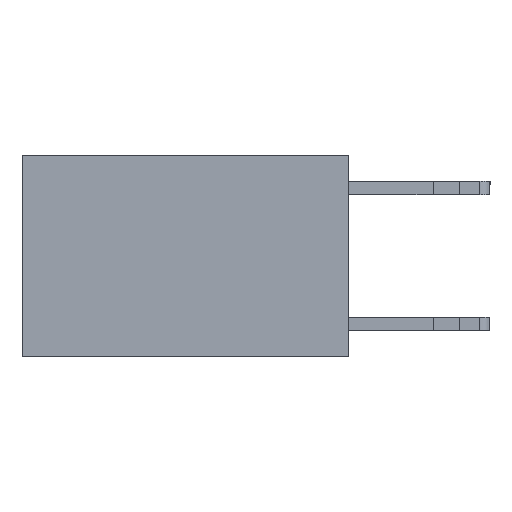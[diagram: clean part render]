
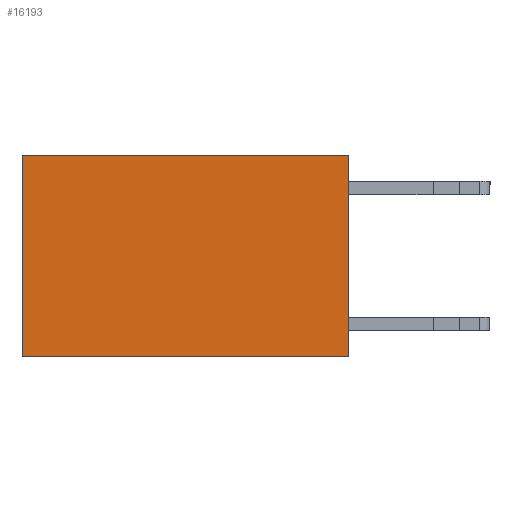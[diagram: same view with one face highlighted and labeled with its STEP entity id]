
A CAD part, left-side view. The second image highlights one B-rep face of the part: STEP entity #16193.
In plain terms, the highlighted planar face has unit normal (-1, 0, 0).
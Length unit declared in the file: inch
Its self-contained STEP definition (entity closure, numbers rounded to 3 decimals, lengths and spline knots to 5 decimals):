
#181 = FACE_OUTER_BOUND ( 'NONE', #7099, .T. ) ;
#214 = DIRECTION ( 'NONE',  ( 0., 1., 0. ) ) ;
#732 = VERTEX_POINT ( 'NONE', #15898 ) ;
#791 = EDGE_CURVE ( 'NONE', #1313, #732, #14803, .T. ) ;
#1313 = VERTEX_POINT ( 'NONE', #6391 ) ;
#1905 = CARTESIAN_POINT ( 'NONE',  ( 0.2625, 0., -0.37 ) ) ;
#4133 = DIRECTION ( 'NONE',  ( 0., 0., -1. ) ) ;
#4247 = LINE ( 'NONE', #9738, #13592 ) ;
#4595 = VECTOR ( 'NONE', #4133, 39.37008 ) ;
#5640 = PLANE ( 'NONE',  #14973 ) ;
#5733 = CARTESIAN_POINT ( 'NONE',  ( 0.2625, 0., 0. ) ) ;
#6015 = EDGE_CURVE ( 'NONE', #7714, #14525, #10716, .T. ) ;
#6265 = EDGE_CURVE ( 'NONE', #7714, #1313, #6900, .T. ) ;
#6391 = CARTESIAN_POINT ( 'NONE',  ( 0.2625, 0.6, 0. ) ) ;
#6900 = LINE ( 'NONE', #12488, #12908 ) ;
#7099 = EDGE_LOOP ( 'NONE', ( #16172, #9218, #14321, #10500 ) ) ;
#7173 = DIRECTION ( 'NONE',  ( 0., 0., -1. ) ) ;
#7268 = DIRECTION ( 'NONE',  ( 1., 0., 0. ) ) ;
#7714 = VERTEX_POINT ( 'NONE', #5733 ) ;
#8097 = CARTESIAN_POINT ( 'NONE',  ( 0.2625, 0.6, 0. ) ) ;
#9218 = ORIENTED_EDGE ( 'NONE', *, *, #10481, .F. ) ;
#9738 = CARTESIAN_POINT ( 'NONE',  ( 0.2625, 0., -0.37 ) ) ;
#10481 = EDGE_CURVE ( 'NONE', #14525, #732, #4247, .T. ) ;
#10500 = ORIENTED_EDGE ( 'NONE', *, *, #6265, .T. ) ;
#10656 = DIRECTION ( 'NONE',  ( 0., 0., -1. ) ) ;
#10716 = LINE ( 'NONE', #17465, #4595 ) ;
#12488 = CARTESIAN_POINT ( 'NONE',  ( 0.2625, 0., 0. ) ) ;
#12908 = VECTOR ( 'NONE', #16815, 39.37008 ) ;
#13592 = VECTOR ( 'NONE', #214, 39.37008 ) ;
#14321 = ORIENTED_EDGE ( 'NONE', *, *, #6015, .F. ) ;
#14525 = VERTEX_POINT ( 'NONE', #1905 ) ;
#14803 = LINE ( 'NONE', #8097, #16113 ) ;
#14973 = AXIS2_PLACEMENT_3D ( 'NONE', #16650, #7268, #7173 ) ;
#15898 = CARTESIAN_POINT ( 'NONE',  ( 0.2625, 0.6, -0.37 ) ) ;
#16113 = VECTOR ( 'NONE', #10656, 39.37008 ) ;
#16172 = ORIENTED_EDGE ( 'NONE', *, *, #791, .T. ) ;
#16193 = ADVANCED_FACE ( 'NONE', ( #181 ), #5640, .F. ) ;
#16650 = CARTESIAN_POINT ( 'NONE',  ( 0.2625, 0., 0. ) ) ;
#16815 = DIRECTION ( 'NONE',  ( 0., 1., 0. ) ) ;
#17465 = CARTESIAN_POINT ( 'NONE',  ( 0.2625, 0., 0. ) ) ;
